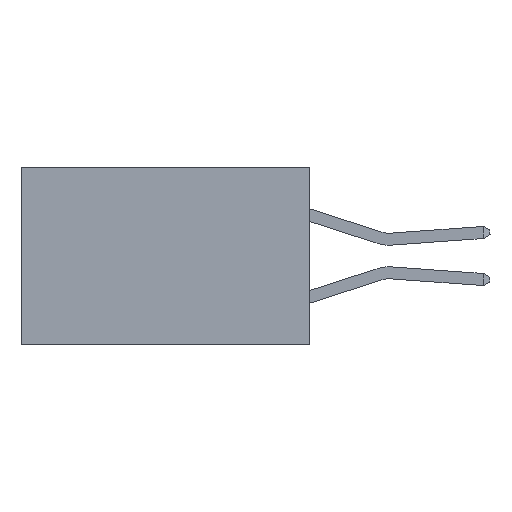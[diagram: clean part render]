
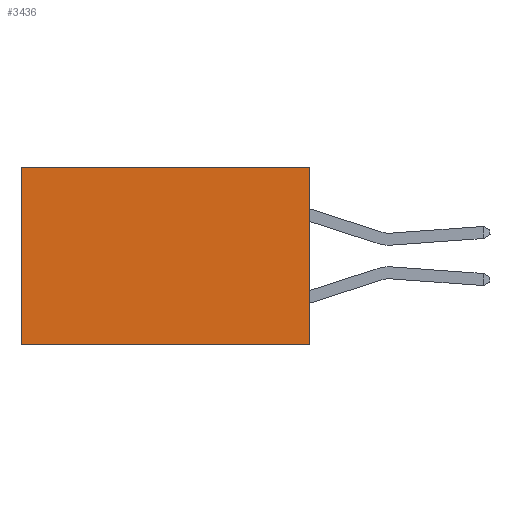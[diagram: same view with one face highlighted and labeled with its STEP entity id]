
A CAD part, left-side view. The second image highlights one B-rep face of the part: STEP entity #3436.
In plain terms, the highlighted planar face has unit normal (-1, 0, 0).
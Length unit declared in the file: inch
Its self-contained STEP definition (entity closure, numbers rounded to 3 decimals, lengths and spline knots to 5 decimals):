
#504 = EDGE_CURVE ( 'NONE', #4954, #5323, #5572, .T. ) ;
#785 = DIRECTION ( 'NONE',  ( 0., 0., -1. ) ) ;
#875 = VECTOR ( 'NONE', #930, 39.37008 ) ;
#930 = DIRECTION ( 'NONE',  ( 0., 0., -1. ) ) ;
#1030 = VERTEX_POINT ( 'NONE', #2620 ) ;
#1139 = VECTOR ( 'NONE', #785, 39.37008 ) ;
#1166 = EDGE_LOOP ( 'NONE', ( #6946, #4772, #2849, #2413 ) ) ;
#1334 = DIRECTION ( 'NONE',  ( 0., 1., 0. ) ) ;
#1999 = LINE ( 'NONE', #3907, #3030 ) ;
#2022 = CARTESIAN_POINT ( 'NONE',  ( 0.2615, 0., -0.37 ) ) ;
#2330 = CARTESIAN_POINT ( 'NONE',  ( 0.2615, 0., -0.37 ) ) ;
#2413 = ORIENTED_EDGE ( 'NONE', *, *, #3546, .T. ) ;
#2469 = CARTESIAN_POINT ( 'NONE',  ( 0.2615, 0., -0.37 ) ) ;
#2620 = CARTESIAN_POINT ( 'NONE',  ( 0.2615, 0., 0. ) ) ;
#2666 = CARTESIAN_POINT ( 'NONE',  ( 0.2615, 0.6, -0.37 ) ) ;
#2713 = VERTEX_POINT ( 'NONE', #5084 ) ;
#2849 = ORIENTED_EDGE ( 'NONE', *, *, #7109, .F. ) ;
#3030 = VECTOR ( 'NONE', #1334, 39.37008 ) ;
#3280 = LINE ( 'NONE', #2022, #1139 ) ;
#3436 = ADVANCED_FACE ( 'NONE', ( #5009 ), #5052, .F. ) ;
#3514 = VECTOR ( 'NONE', #8137, 39.37008 ) ;
#3546 = EDGE_CURVE ( 'NONE', #1030, #2713, #1999, .T. ) ;
#3784 = DIRECTION ( 'NONE',  ( 1., 0., 0. ) ) ;
#3793 = CARTESIAN_POINT ( 'NONE',  ( 0.2615, 0., -0.37 ) ) ;
#3907 = CARTESIAN_POINT ( 'NONE',  ( 0.2615, 0., 0. ) ) ;
#4518 = AXIS2_PLACEMENT_3D ( 'NONE', #2469, #3784, #7713 ) ;
#4772 = ORIENTED_EDGE ( 'NONE', *, *, #504, .F. ) ;
#4800 = LINE ( 'NONE', #8125, #875 ) ;
#4954 = VERTEX_POINT ( 'NONE', #2330 ) ;
#5009 = FACE_OUTER_BOUND ( 'NONE', #1166, .T. ) ;
#5052 = PLANE ( 'NONE',  #4518 ) ;
#5084 = CARTESIAN_POINT ( 'NONE',  ( 0.2615, 0.6, 0. ) ) ;
#5323 = VERTEX_POINT ( 'NONE', #2666 ) ;
#5572 = LINE ( 'NONE', #3793, #3514 ) ;
#6463 = EDGE_CURVE ( 'NONE', #2713, #5323, #4800, .T. ) ;
#6946 = ORIENTED_EDGE ( 'NONE', *, *, #6463, .T. ) ;
#7109 = EDGE_CURVE ( 'NONE', #1030, #4954, #3280, .T. ) ;
#7713 = DIRECTION ( 'NONE',  ( 0., 0., -1. ) ) ;
#8125 = CARTESIAN_POINT ( 'NONE',  ( 0.2615, 0.6, -0.37 ) ) ;
#8137 = DIRECTION ( 'NONE',  ( 0., 1., 0. ) ) ;
